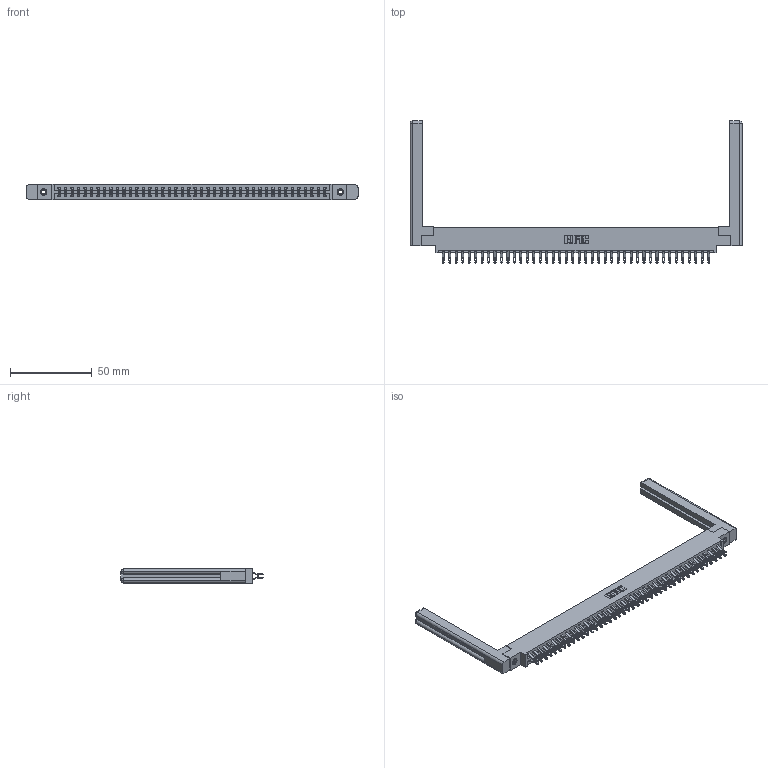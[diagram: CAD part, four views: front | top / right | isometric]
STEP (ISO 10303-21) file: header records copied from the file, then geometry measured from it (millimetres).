
FILE_DESCRIPTION (( 'STEP AP203' ), '1' );
FILE_NAME ('387-084-555-858.STEP', '2019-10-23T02:02:24', ( '' ), ( '' ), 'SwSTEP 2.0', 'SolidWorks 2016', '' );
FILE_SCHEMA (( 'CONFIG_CONTROL_DESIGN' ));
Length unit declared in the file: inch
Products named in the file (5): 345-250-001_345-250-001-102; 307-220-058; 337 Part_0.170 Offset - 0.156 Dia-TI; 387-084-555-858; 345-292-001_555 Tail
Assembly tree (89 placements, depth 2):
  387-084-555-858
    337 Part_0.170 Offset - 0.156 Dia-TI
    345-292-001_555 Tail  x84
    345-250-001_345-250-001-102  x2
    307-220-058  x2
Bounding box: 203.05 x 86.87 x 9.4 mm (x, y, z)
Volume: 28667.3 mm3; surface area: 30406.7 mm2
Topology: 89 solids, 89 shells, 5300 faces, 16553 edges, 11022 vertices
Faces by surface type: plane 3182, cylinder 2094, cone 12, torus 12
Entity records: 35656 total; most frequent: CARTESIAN_POINT 6051, ORIENTED_EDGE 5896, DIRECTION 5132, EDGE_CURVE 2948, LINE 2752, VECTOR 2752, VERTEX_POINT 1958, AXIS2_PLACEMENT_3D 1190
